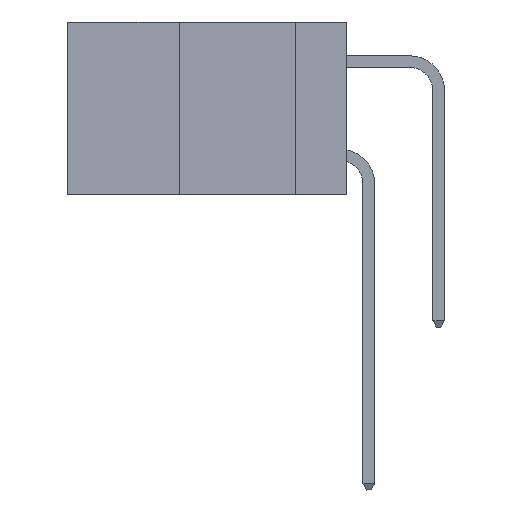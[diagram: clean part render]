
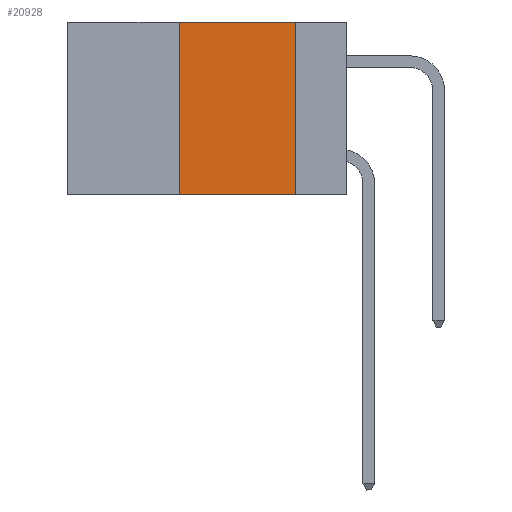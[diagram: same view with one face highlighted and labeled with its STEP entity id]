
A CAD part, left-side view. The second image highlights one B-rep face of the part: STEP entity #20928.
In plain terms, the highlighted planar face has unit normal (-1, 0, 0).
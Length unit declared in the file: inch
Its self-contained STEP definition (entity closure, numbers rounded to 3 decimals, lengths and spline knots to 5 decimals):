
#200 = ORIENTED_EDGE ( 'NONE', *, *, #23349, .F. ) ;
#1679 = EDGE_LOOP ( 'NONE', ( #200, #4230, #17273, #18387 ) ) ;
#4230 = ORIENTED_EDGE ( 'NONE', *, *, #4675, .F. ) ;
#4675 = EDGE_CURVE ( 'NONE', #8735, #19640, #7598, .T. ) ;
#5124 = CARTESIAN_POINT ( 'NONE',  ( 0., 0.11, -0.37 ) ) ;
#6360 = VECTOR ( 'NONE', #8146, 39.37008 ) ;
#6907 = DIRECTION ( 'NONE',  ( 0., 0., 1. ) ) ;
#7598 = LINE ( 'NONE', #11576, #6360 ) ;
#7981 = FACE_OUTER_BOUND ( 'NONE', #1679, .T. ) ;
#8146 = DIRECTION ( 'NONE',  ( 0., -1., 0. ) ) ;
#8151 = LINE ( 'NONE', #25121, #15311 ) ;
#8212 = DIRECTION ( 'NONE',  ( 0., 0., -1. ) ) ;
#8483 = PLANE ( 'NONE',  #10156 ) ;
#8735 = VERTEX_POINT ( 'NONE', #18766 ) ;
#9673 = EDGE_CURVE ( 'NONE', #23511, #23000, #8151, .T. ) ;
#10156 = AXIS2_PLACEMENT_3D ( 'NONE', #22462, #20564, #24420 ) ;
#10720 = CARTESIAN_POINT ( 'NONE',  ( 0., 0.36, 0. ) ) ;
#11576 = CARTESIAN_POINT ( 'NONE',  ( 0., 0.6, 0. ) ) ;
#13301 = DIRECTION ( 'NONE',  ( 0., -1., 0. ) ) ;
#13817 = VECTOR ( 'NONE', #8212, 39.37008 ) ;
#14201 = CARTESIAN_POINT ( 'NONE',  ( 0., 0.36, -0.37 ) ) ;
#14859 = EDGE_CURVE ( 'NONE', #23511, #8735, #16162, .T. ) ;
#15311 = VECTOR ( 'NONE', #13301, 39.37008 ) ;
#16162 = LINE ( 'NONE', #10720, #17414 ) ;
#17273 = ORIENTED_EDGE ( 'NONE', *, *, #14859, .F. ) ;
#17414 = VECTOR ( 'NONE', #6907, 39.37008 ) ;
#18387 = ORIENTED_EDGE ( 'NONE', *, *, #9673, .T. ) ;
#18766 = CARTESIAN_POINT ( 'NONE',  ( 0., 0.36, 0. ) ) ;
#19640 = VERTEX_POINT ( 'NONE', #21012 ) ;
#20564 = DIRECTION ( 'NONE',  ( 1., 0., 0. ) ) ;
#20928 = ADVANCED_FACE ( 'NONE', ( #7981 ), #8483, .F. ) ;
#21012 = CARTESIAN_POINT ( 'NONE',  ( 0., 0.11, 0. ) ) ;
#22021 = CARTESIAN_POINT ( 'NONE',  ( 0., 0.11, 0. ) ) ;
#22462 = CARTESIAN_POINT ( 'NONE',  ( 0., 0.6, 0. ) ) ;
#22739 = LINE ( 'NONE', #22021, #13817 ) ;
#23000 = VERTEX_POINT ( 'NONE', #5124 ) ;
#23349 = EDGE_CURVE ( 'NONE', #19640, #23000, #22739, .T. ) ;
#23511 = VERTEX_POINT ( 'NONE', #14201 ) ;
#24420 = DIRECTION ( 'NONE',  ( 0., 0., -1. ) ) ;
#25121 = CARTESIAN_POINT ( 'NONE',  ( 0., 0.6, -0.37 ) ) ;
